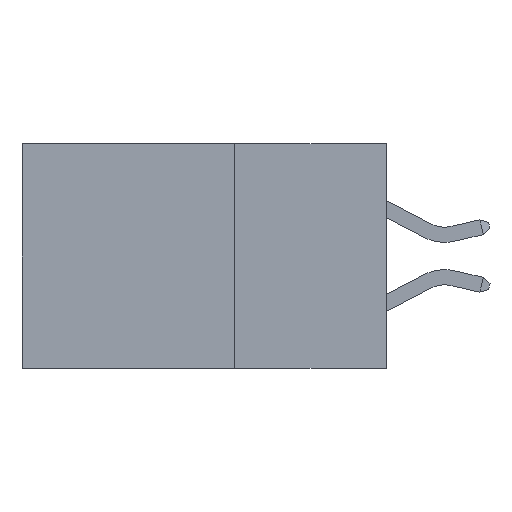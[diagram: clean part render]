
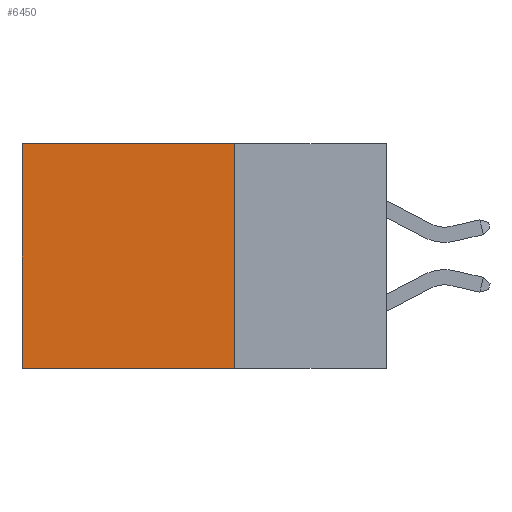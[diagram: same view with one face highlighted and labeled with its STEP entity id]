
A CAD part, left-side view. The second image highlights one B-rep face of the part: STEP entity #6450.
In plain terms, the highlighted planar face has unit normal (-1, 0, 0).
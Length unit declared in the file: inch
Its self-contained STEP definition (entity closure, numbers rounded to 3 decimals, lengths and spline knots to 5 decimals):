
#12 = VECTOR ( 'NONE', #12228, 39.37008 ) ;
#137 = ORIENTED_EDGE ( 'NONE', *, *, #9249, .T. ) ;
#269 = VECTOR ( 'NONE', #896, 39.37008 ) ;
#428 = ORIENTED_EDGE ( 'NONE', *, *, #1293, .F. ) ;
#637 = DIRECTION ( 'NONE',  ( 1., 0., 0. ) ) ;
#756 = VERTEX_POINT ( 'NONE', #9758 ) ;
#896 = DIRECTION ( 'NONE',  ( 0., 0., -1. ) ) ;
#1291 = FACE_OUTER_BOUND ( 'NONE', #3214, .T. ) ;
#1293 = EDGE_CURVE ( 'NONE', #8414, #9385, #5401, .T. ) ;
#1946 = AXIS2_PLACEMENT_3D ( 'NONE', #6725, #637, #7712 ) ;
#2070 = CARTESIAN_POINT ( 'NONE',  ( 0.2615, 0.6, 0. ) ) ;
#2258 = VERTEX_POINT ( 'NONE', #2070 ) ;
#2701 = VECTOR ( 'NONE', #5552, 39.37008 ) ;
#3214 = EDGE_LOOP ( 'NONE', ( #137, #428, #8546, #10616 ) ) ;
#3492 = LINE ( 'NONE', #3732, #11220 ) ;
#3732 = CARTESIAN_POINT ( 'NONE',  ( 0.2615, 0.25, -0.37 ) ) ;
#4218 = CARTESIAN_POINT ( 'NONE',  ( 0.2615, 0.25, 0. ) ) ;
#4751 = DIRECTION ( 'NONE',  ( 0., 0., -1. ) ) ;
#5401 = LINE ( 'NONE', #10537, #2701 ) ;
#5552 = DIRECTION ( 'NONE',  ( 0., 1., 0. ) ) ;
#5642 = PLANE ( 'NONE',  #1946 ) ;
#6317 = CARTESIAN_POINT ( 'NONE',  ( 0.2615, 0.6, -0.37 ) ) ;
#6450 = ADVANCED_FACE ( 'NONE', ( #1291 ), #5642, .F. ) ;
#6725 = CARTESIAN_POINT ( 'NONE',  ( 0.2615, 0.25, -0.37 ) ) ;
#7145 = EDGE_CURVE ( 'NONE', #756, #8414, #3492, .T. ) ;
#7481 = EDGE_CURVE ( 'NONE', #756, #2258, #10454, .T. ) ;
#7712 = DIRECTION ( 'NONE',  ( 0., 0., -1. ) ) ;
#8414 = VERTEX_POINT ( 'NONE', #12644 ) ;
#8546 = ORIENTED_EDGE ( 'NONE', *, *, #7145, .F. ) ;
#9249 = EDGE_CURVE ( 'NONE', #2258, #9385, #11005, .T. ) ;
#9385 = VERTEX_POINT ( 'NONE', #6317 ) ;
#9758 = CARTESIAN_POINT ( 'NONE',  ( 0.2615, 0.25, 0. ) ) ;
#10454 = LINE ( 'NONE', #4218, #12 ) ;
#10537 = CARTESIAN_POINT ( 'NONE',  ( 0.2615, 0.25, -0.37 ) ) ;
#10616 = ORIENTED_EDGE ( 'NONE', *, *, #7481, .T. ) ;
#11005 = LINE ( 'NONE', #12931, #269 ) ;
#11220 = VECTOR ( 'NONE', #4751, 39.37008 ) ;
#12228 = DIRECTION ( 'NONE',  ( 0., 1., 0. ) ) ;
#12644 = CARTESIAN_POINT ( 'NONE',  ( 0.2615, 0.25, -0.37 ) ) ;
#12931 = CARTESIAN_POINT ( 'NONE',  ( 0.2615, 0.6, -0.37 ) ) ;
